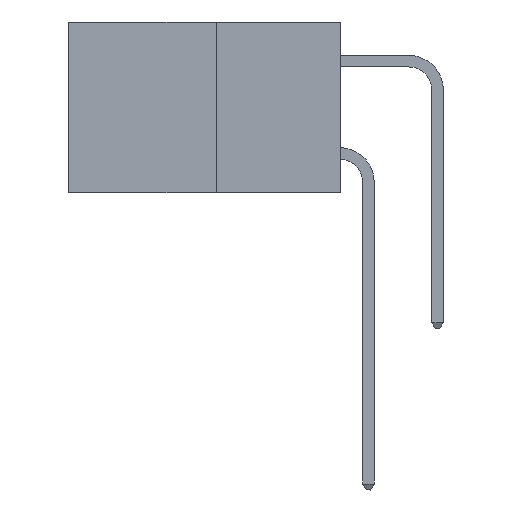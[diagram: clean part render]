
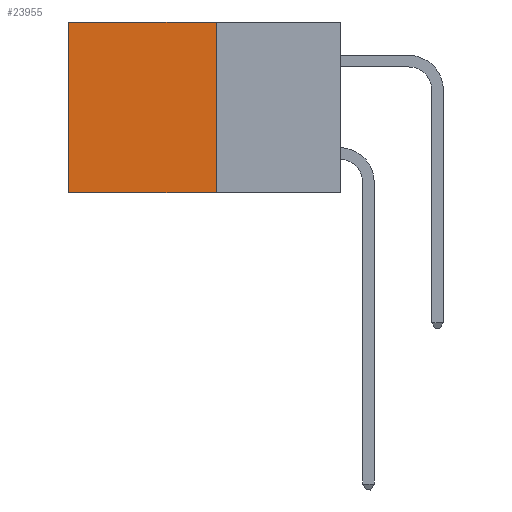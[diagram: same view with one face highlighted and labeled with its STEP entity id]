
A CAD part, left-side view. The second image highlights one B-rep face of the part: STEP entity #23955.
In plain terms, the highlighted planar face has unit normal (-1, 0, 0).
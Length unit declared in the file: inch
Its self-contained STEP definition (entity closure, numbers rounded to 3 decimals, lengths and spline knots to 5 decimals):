
#2736 = PLANE ( 'NONE',  #7824 ) ;
#3500 = EDGE_CURVE ( 'NONE', #19468, #4320, #12284, .T. ) ;
#3600 = EDGE_CURVE ( 'NONE', #18259, #28704, #20819, .T. ) ;
#4196 = ORIENTED_EDGE ( 'NONE', *, *, #3600, .T. ) ;
#4320 = VERTEX_POINT ( 'NONE', #4385 ) ;
#4385 = CARTESIAN_POINT ( 'NONE',  ( 0.277, 0.27, -0.37 ) ) ;
#5217 = DIRECTION ( 'NONE',  ( 0., 0., -1. ) ) ;
#6661 = VECTOR ( 'NONE', #25005, 39.37008 ) ;
#7645 = CARTESIAN_POINT ( 'NONE',  ( 0.277, 0.27, -0.37 ) ) ;
#7824 = AXIS2_PLACEMENT_3D ( 'NONE', #29819, #19982, #5217 ) ;
#9036 = CARTESIAN_POINT ( 'NONE',  ( 0.277, 0.27, 0. ) ) ;
#9977 = EDGE_CURVE ( 'NONE', #19468, #18259, #17190, .T. ) ;
#10234 = FACE_OUTER_BOUND ( 'NONE', #20533, .T. ) ;
#11380 = VECTOR ( 'NONE', #26333, 39.37008 ) ;
#12284 = LINE ( 'NONE', #23660, #29721 ) ;
#12287 = CARTESIAN_POINT ( 'NONE',  ( 0.277, 0.59, 0. ) ) ;
#14983 = VECTOR ( 'NONE', #20600, 39.37008 ) ;
#16264 = ORIENTED_EDGE ( 'NONE', *, *, #3500, .F. ) ;
#16358 = ORIENTED_EDGE ( 'NONE', *, *, #9977, .T. ) ;
#17190 = LINE ( 'NONE', #9036, #11380 ) ;
#17668 = ORIENTED_EDGE ( 'NONE', *, *, #27138, .F. ) ;
#18259 = VERTEX_POINT ( 'NONE', #12287 ) ;
#19468 = VERTEX_POINT ( 'NONE', #26964 ) ;
#19802 = LINE ( 'NONE', #7645, #6661 ) ;
#19982 = DIRECTION ( 'NONE',  ( 1., 0., 0. ) ) ;
#20533 = EDGE_LOOP ( 'NONE', ( #4196, #17668, #16264, #16358 ) ) ;
#20600 = DIRECTION ( 'NONE',  ( 0., 0., -1. ) ) ;
#20733 = CARTESIAN_POINT ( 'NONE',  ( 0.277, 0.59, -0.37 ) ) ;
#20819 = LINE ( 'NONE', #20733, #14983 ) ;
#23660 = CARTESIAN_POINT ( 'NONE',  ( 0.277, 0.27, -0.37 ) ) ;
#23724 = DIRECTION ( 'NONE',  ( 0., 0., -1. ) ) ;
#23955 = ADVANCED_FACE ( 'NONE', ( #10234 ), #2736, .F. ) ;
#25005 = DIRECTION ( 'NONE',  ( 0., 1., 0. ) ) ;
#25579 = CARTESIAN_POINT ( 'NONE',  ( 0.277, 0.59, -0.37 ) ) ;
#26333 = DIRECTION ( 'NONE',  ( 0., 1., 0. ) ) ;
#26964 = CARTESIAN_POINT ( 'NONE',  ( 0.277, 0.27, 0. ) ) ;
#27138 = EDGE_CURVE ( 'NONE', #4320, #28704, #19802, .T. ) ;
#28704 = VERTEX_POINT ( 'NONE', #25579 ) ;
#29721 = VECTOR ( 'NONE', #23724, 39.37008 ) ;
#29819 = CARTESIAN_POINT ( 'NONE',  ( 0.277, 0.27, -0.37 ) ) ;
